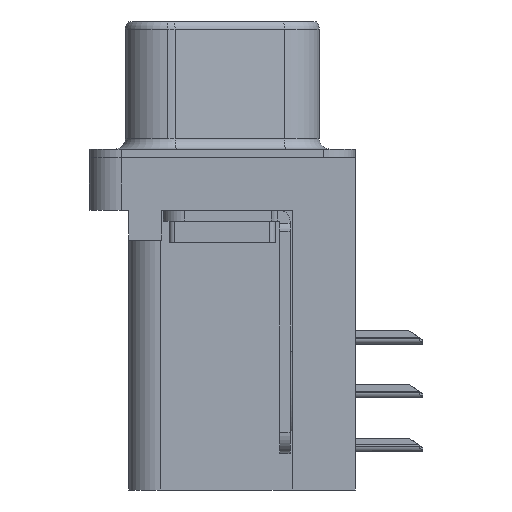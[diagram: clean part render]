
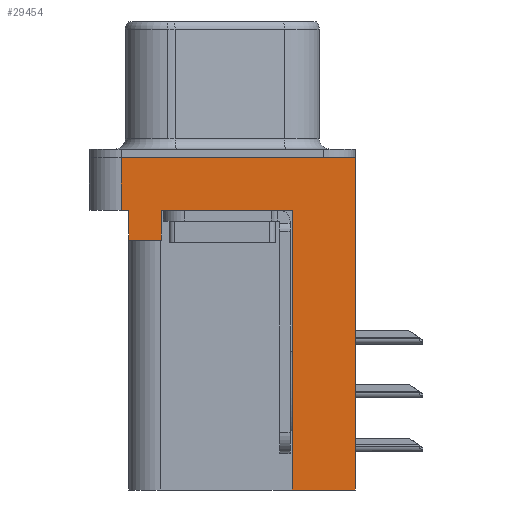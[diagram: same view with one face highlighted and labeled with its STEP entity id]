
A CAD part, left-side view. The second image highlights one B-rep face of the part: STEP entity #29454.
In plain terms, the highlighted planar face has unit normal (-1, 0, 0).
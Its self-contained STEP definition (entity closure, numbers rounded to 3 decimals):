
#150 = CARTESIAN_POINT ( 'NONE',  ( -3., -6.275, 0. ) ) ;
#228 = VECTOR ( 'NONE', #7038, 1000. ) ;
#318 = CARTESIAN_POINT ( 'NONE',  ( -3., 4.425, -2.5 ) ) ;
#391 = DIRECTION ( 'NONE',  ( 0., 0., 1. ) ) ;
#644 = VECTOR ( 'NONE', #19327, 1000. ) ;
#856 = VERTEX_POINT ( 'NONE', #21960 ) ;
#883 = CARTESIAN_POINT ( 'NONE',  ( -3., -6.275, -2.5 ) ) ;
#1217 = VECTOR ( 'NONE', #29478, 1000. ) ;
#1419 = LINE ( 'NONE', #2286, #644 ) ;
#1985 = EDGE_CURVE ( 'NONE', #23504, #24321, #16930, .T. ) ;
#2286 = CARTESIAN_POINT ( 'NONE',  ( -3., -6.275, 0. ) ) ;
#2392 = EDGE_CURVE ( 'NONE', #856, #23504, #25465, .T. ) ;
#2800 = VECTOR ( 'NONE', #22426, 1000. ) ;
#3308 = LINE ( 'NONE', #16381, #27567 ) ;
#3522 = ORIENTED_EDGE ( 'NONE', *, *, #20161, .T. ) ;
#4132 = VECTOR ( 'NONE', #7796, 1000. ) ;
#4146 = DIRECTION ( 'NONE',  ( 0., 1., 0. ) ) ;
#4408 = AXIS2_PLACEMENT_3D ( 'NONE', #12689, #15102, #391 ) ;
#4873 = CARTESIAN_POINT ( 'NONE',  ( -3., -3.295, -15.7 ) ) ;
#5590 = ORIENTED_EDGE ( 'NONE', *, *, #14797, .F. ) ;
#6288 = CARTESIAN_POINT ( 'NONE',  ( -3., 4.425, -3.9 ) ) ;
#6570 = EDGE_CURVE ( 'NONE', #6625, #30079, #1419, .T. ) ;
#6625 = VERTEX_POINT ( 'NONE', #21956 ) ;
#7038 = DIRECTION ( 'NONE',  ( 0., -1., 0. ) ) ;
#7796 = DIRECTION ( 'NONE',  ( 0., 0., 1. ) ) ;
#8187 = EDGE_CURVE ( 'NONE', #16296, #6625, #11034, .T. ) ;
#8610 = LINE ( 'NONE', #15967, #27099 ) ;
#8913 = CARTESIAN_POINT ( 'NONE',  ( -3., 4.425, -3.9 ) ) ;
#9057 = ORIENTED_EDGE ( 'NONE', *, *, #2392, .T. ) ;
#9373 = LINE ( 'NONE', #24924, #2800 ) ;
#9857 = EDGE_CURVE ( 'NONE', #17526, #30915, #8610, .T. ) ;
#10189 = PLANE ( 'NONE',  #4408 ) ;
#10853 = ORIENTED_EDGE ( 'NONE', *, *, #1985, .T. ) ;
#11034 = LINE ( 'NONE', #30190, #29481 ) ;
#11064 = CARTESIAN_POINT ( 'NONE',  ( -3., -6.275, -15.7 ) ) ;
#12689 = CARTESIAN_POINT ( 'NONE',  ( -3., -6.275, -2.5 ) ) ;
#13647 = DIRECTION ( 'NONE',  ( 0., -1., 0. ) ) ;
#14797 = EDGE_CURVE ( 'NONE', #18696, #24321, #30680, .T. ) ;
#15102 = DIRECTION ( 'NONE',  ( -1., 0., 0. ) ) ;
#15827 = DIRECTION ( 'NONE',  ( 0., 0., 1. ) ) ;
#15967 = CARTESIAN_POINT ( 'NONE',  ( -3., 4.425, -3.9 ) ) ;
#16296 = VERTEX_POINT ( 'NONE', #30313 ) ;
#16381 = CARTESIAN_POINT ( 'NONE',  ( -3., -3.295, -15.7 ) ) ;
#16930 = LINE ( 'NONE', #883, #28923 ) ;
#17526 = VERTEX_POINT ( 'NONE', #8913 ) ;
#17672 = VERTEX_POINT ( 'NONE', #11064 ) ;
#18696 = VERTEX_POINT ( 'NONE', #4873 ) ;
#18906 = CARTESIAN_POINT ( 'NONE',  ( -3., -6.275, -2.5 ) ) ;
#19327 = DIRECTION ( 'NONE',  ( 0., -1., 0. ) ) ;
#19568 = EDGE_CURVE ( 'NONE', #17672, #18696, #3308, .T. ) ;
#19659 = LINE ( 'NONE', #18906, #228 ) ;
#20161 = EDGE_CURVE ( 'NONE', #16296, #30915, #19659, .T. ) ;
#20815 = ORIENTED_EDGE ( 'NONE', *, *, #25358, .T. ) ;
#21956 = CARTESIAN_POINT ( 'NONE',  ( -3., 4.775, 0. ) ) ;
#21960 = CARTESIAN_POINT ( 'NONE',  ( -3., 2.895, -3.9 ) ) ;
#22426 = DIRECTION ( 'NONE',  ( 0., 0., 1. ) ) ;
#23187 = DIRECTION ( 'NONE',  ( 0., 1., 0. ) ) ;
#23504 = VERTEX_POINT ( 'NONE', #30660 ) ;
#24321 = VERTEX_POINT ( 'NONE', #26141 ) ;
#24686 = CARTESIAN_POINT ( 'NONE',  ( -3., -3.295, -15.7 ) ) ;
#24924 = CARTESIAN_POINT ( 'NONE',  ( -3., -6.275, -2.5 ) ) ;
#24970 = ORIENTED_EDGE ( 'NONE', *, *, #19568, .F. ) ;
#25236 = EDGE_LOOP ( 'NONE', ( #26541, #25797, #3522, #31360, #30096, #9057, #10853, #5590, #24970, #20815 ) ) ;
#25312 = CARTESIAN_POINT ( 'NONE',  ( -3., 2.895, -3.9 ) ) ;
#25358 = EDGE_CURVE ( 'NONE', #17672, #30079, #9373, .T. ) ;
#25465 = LINE ( 'NONE', #25312, #1217 ) ;
#25797 = ORIENTED_EDGE ( 'NONE', *, *, #8187, .F. ) ;
#26141 = CARTESIAN_POINT ( 'NONE',  ( -3., -3.295, -2.5 ) ) ;
#26541 = ORIENTED_EDGE ( 'NONE', *, *, #6570, .F. ) ;
#27099 = VECTOR ( 'NONE', #30439, 1000. ) ;
#27185 = EDGE_CURVE ( 'NONE', #856, #17526, #30400, .T. ) ;
#27567 = VECTOR ( 'NONE', #4146, 1000. ) ;
#28773 = FACE_OUTER_BOUND ( 'NONE', #25236, .T. ) ;
#28923 = VECTOR ( 'NONE', #13647, 1000. ) ;
#29454 = ADVANCED_FACE ( 'NONE', ( #28773 ), #10189, .T. ) ;
#29478 = DIRECTION ( 'NONE',  ( 0., 0., 1. ) ) ;
#29481 = VECTOR ( 'NONE', #15827, 1000. ) ;
#30079 = VERTEX_POINT ( 'NONE', #150 ) ;
#30096 = ORIENTED_EDGE ( 'NONE', *, *, #27185, .F. ) ;
#30190 = CARTESIAN_POINT ( 'NONE',  ( -3., 4.775, -2.5 ) ) ;
#30313 = CARTESIAN_POINT ( 'NONE',  ( -3., 4.775, -2.5 ) ) ;
#30400 = LINE ( 'NONE', #6288, #31163 ) ;
#30439 = DIRECTION ( 'NONE',  ( 0., 0., 1. ) ) ;
#30660 = CARTESIAN_POINT ( 'NONE',  ( -3., 2.895, -2.5 ) ) ;
#30680 = LINE ( 'NONE', #24686, #4132 ) ;
#30915 = VERTEX_POINT ( 'NONE', #318 ) ;
#31163 = VECTOR ( 'NONE', #23187, 1000. ) ;
#31360 = ORIENTED_EDGE ( 'NONE', *, *, #9857, .F. ) ;
